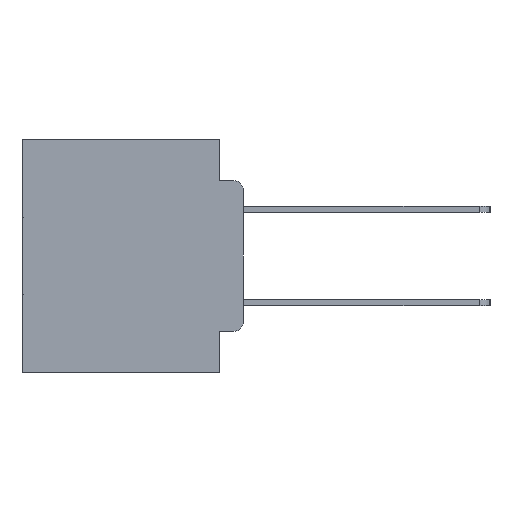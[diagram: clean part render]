
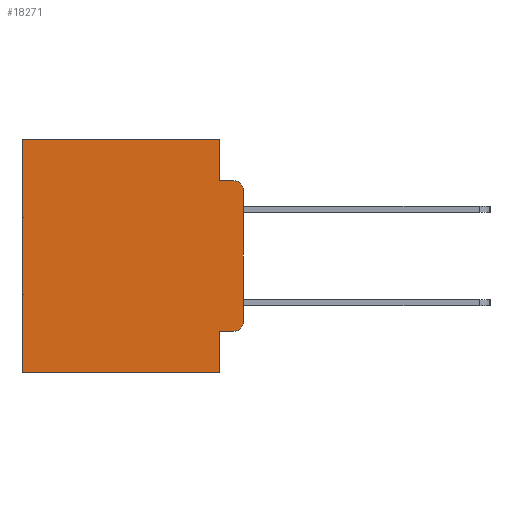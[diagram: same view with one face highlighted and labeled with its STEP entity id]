
A CAD part, left-side view. The second image highlights one B-rep face of the part: STEP entity #18271.
In plain terms, the highlighted planar face has unit normal (-1, 0, 0).
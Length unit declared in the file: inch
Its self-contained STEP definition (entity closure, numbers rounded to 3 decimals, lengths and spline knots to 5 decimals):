
#10 = DIRECTION ( 'NONE',  ( 0., 0., -1. ) ) ;
#152 = EDGE_CURVE ( 'NONE', #9563, #14871, #5240, .T. ) ;
#1218 = EDGE_CURVE ( 'NONE', #31943, #27119, #18344, .T. ) ;
#1220 = LINE ( 'NONE', #25572, #20149 ) ;
#1717 = CARTESIAN_POINT ( 'NONE',  ( 0.298, 0.473, -0.5 ) ) ;
#1939 = CARTESIAN_POINT ( 'NONE',  ( 0.298, 0., 0. ) ) ;
#2114 = DIRECTION ( 'NONE',  ( 0., -1., 0. ) ) ;
#2379 = VERTEX_POINT ( 'NONE', #3986 ) ;
#2478 = CARTESIAN_POINT ( 'NONE',  ( 0.298, 0.051, -0.0885 ) ) ;
#2847 = CARTESIAN_POINT ( 'NONE',  ( 0.298, 0.02, -0.0885 ) ) ;
#3167 = VERTEX_POINT ( 'NONE', #4588 ) ;
#3423 = CARTESIAN_POINT ( 'NONE',  ( 0.298, 0.051, 0. ) ) ;
#3986 = CARTESIAN_POINT ( 'NONE',  ( 0.298, 0.051, -0.0885 ) ) ;
#4492 = EDGE_CURVE ( 'NONE', #2379, #22608, #4625, .T. ) ;
#4588 = CARTESIAN_POINT ( 'NONE',  ( 0.298, 0.051, 0. ) ) ;
#4625 = LINE ( 'NONE', #2478, #17025 ) ;
#5240 = LINE ( 'NONE', #8095, #16857 ) ;
#5512 = EDGE_CURVE ( 'NONE', #27119, #14871, #12323, .T. ) ;
#5809 = VECTOR ( 'NONE', #16875, 39.37008 ) ;
#6748 = DIRECTION ( 'NONE',  ( -1., 0., 0. ) ) ;
#7572 = DIRECTION ( 'NONE',  ( 0., -1., 0. ) ) ;
#7820 = VECTOR ( 'NONE', #28628, 39.37008 ) ;
#8084 = CARTESIAN_POINT ( 'NONE',  ( 0.298, 0., 0. ) ) ;
#8095 = CARTESIAN_POINT ( 'NONE',  ( 0.298, 0., 0. ) ) ;
#8290 = DIRECTION ( 'NONE',  ( 0., 1., 0. ) ) ;
#9064 = EDGE_CURVE ( 'NONE', #12530, #10380, #1220, .T. ) ;
#9485 = CARTESIAN_POINT ( 'NONE',  ( 0.298, 0.051, -0.4115 ) ) ;
#9563 = VERTEX_POINT ( 'NONE', #10858 ) ;
#10147 = DIRECTION ( 'NONE',  ( 0., 0., -1. ) ) ;
#10236 = ORIENTED_EDGE ( 'NONE', *, *, #30087, .T. ) ;
#10261 = ORIENTED_EDGE ( 'NONE', *, *, #1218, .T. ) ;
#10380 = VERTEX_POINT ( 'NONE', #1717 ) ;
#10473 = EDGE_CURVE ( 'NONE', #3167, #2379, #21031, .T. ) ;
#10565 = DIRECTION ( 'NONE',  ( 0., 0., -1. ) ) ;
#10858 = CARTESIAN_POINT ( 'NONE',  ( 0.298, 0., -0.1085 ) ) ;
#11286 = ORIENTED_EDGE ( 'NONE', *, *, #30655, .F. ) ;
#11836 = VECTOR ( 'NONE', #2114, 39.37008 ) ;
#12239 = ORIENTED_EDGE ( 'NONE', *, *, #30223, .T. ) ;
#12323 = CIRCLE ( 'NONE', #19967, 0.02 ) ;
#12423 = LINE ( 'NONE', #1939, #5809 ) ;
#12530 = VERTEX_POINT ( 'NONE', #28434 ) ;
#14271 = ORIENTED_EDGE ( 'NONE', *, *, #9064, .F. ) ;
#14494 = DIRECTION ( 'NONE',  ( 0., 0., -1. ) ) ;
#14855 = DIRECTION ( 'NONE',  ( -1., 0., 0. ) ) ;
#14871 = VERTEX_POINT ( 'NONE', #15577 ) ;
#15054 = ORIENTED_EDGE ( 'NONE', *, *, #4492, .F. ) ;
#15540 = FACE_OUTER_BOUND ( 'NONE', #27481, .T. ) ;
#15577 = CARTESIAN_POINT ( 'NONE',  ( 0.298, 0., -0.3915 ) ) ;
#15877 = DIRECTION ( 'NONE',  ( 0., 0., -1. ) ) ;
#16571 = AXIS2_PLACEMENT_3D ( 'NONE', #29612, #14855, #10 ) ;
#16857 = VECTOR ( 'NONE', #10147, 39.37008 ) ;
#16875 = DIRECTION ( 'NONE',  ( 0., 1., 0. ) ) ;
#17025 = VECTOR ( 'NONE', #7572, 39.37008 ) ;
#18271 = ADVANCED_FACE ( 'NONE', ( #15540 ), #30190, .F. ) ;
#18344 = LINE ( 'NONE', #9485, #11836 ) ;
#19030 = CIRCLE ( 'NONE', #16571, 0.02 ) ;
#19123 = ORIENTED_EDGE ( 'NONE', *, *, #10473, .F. ) ;
#19375 = ORIENTED_EDGE ( 'NONE', *, *, #5512, .T. ) ;
#19692 = VECTOR ( 'NONE', #15877, 39.37008 ) ;
#19967 = AXIS2_PLACEMENT_3D ( 'NONE', #21533, #6748, #24013 ) ;
#20149 = VECTOR ( 'NONE', #8290, 39.37008 ) ;
#20248 = VECTOR ( 'NONE', #14494, 39.37008 ) ;
#20484 = LINE ( 'NONE', #3423, #19692 ) ;
#20644 = CARTESIAN_POINT ( 'NONE',  ( 0.298, 0.051, -0.4115 ) ) ;
#20947 = LINE ( 'NONE', #26169, #7820 ) ;
#21031 = LINE ( 'NONE', #21808, #20248 ) ;
#21533 = CARTESIAN_POINT ( 'NONE',  ( 0.298, 0.02, -0.3915 ) ) ;
#21808 = CARTESIAN_POINT ( 'NONE',  ( 0.298, 0.051, 0. ) ) ;
#22608 = VERTEX_POINT ( 'NONE', #2847 ) ;
#24013 = DIRECTION ( 'NONE',  ( 0., 0., -1. ) ) ;
#24658 = EDGE_CURVE ( 'NONE', #9563, #22608, #19030, .T. ) ;
#25358 = DIRECTION ( 'NONE',  ( 1., 0., 0. ) ) ;
#25572 = CARTESIAN_POINT ( 'NONE',  ( 0.298, 0., -0.5 ) ) ;
#26169 = CARTESIAN_POINT ( 'NONE',  ( 0.298, 0.473, 0. ) ) ;
#27119 = VERTEX_POINT ( 'NONE', #28186 ) ;
#27481 = EDGE_LOOP ( 'NONE', ( #27916, #30423, #15054, #19123, #12239, #10236, #14271, #11286, #10261, #19375 ) ) ;
#27916 = ORIENTED_EDGE ( 'NONE', *, *, #152, .F. ) ;
#28186 = CARTESIAN_POINT ( 'NONE',  ( 0.298, 0.02, -0.4115 ) ) ;
#28434 = CARTESIAN_POINT ( 'NONE',  ( 0.298, 0.051, -0.5 ) ) ;
#28628 = DIRECTION ( 'NONE',  ( 0., 0., -1. ) ) ;
#29211 = VERTEX_POINT ( 'NONE', #31293 ) ;
#29612 = CARTESIAN_POINT ( 'NONE',  ( 0.298, 0.02, -0.1085 ) ) ;
#30087 = EDGE_CURVE ( 'NONE', #29211, #10380, #20947, .T. ) ;
#30190 = PLANE ( 'NONE',  #30674 ) ;
#30223 = EDGE_CURVE ( 'NONE', #3167, #29211, #12423, .T. ) ;
#30423 = ORIENTED_EDGE ( 'NONE', *, *, #24658, .T. ) ;
#30655 = EDGE_CURVE ( 'NONE', #31943, #12530, #20484, .T. ) ;
#30674 = AXIS2_PLACEMENT_3D ( 'NONE', #8084, #25358, #10565 ) ;
#31293 = CARTESIAN_POINT ( 'NONE',  ( 0.298, 0.473, 0. ) ) ;
#31943 = VERTEX_POINT ( 'NONE', #20644 ) ;
